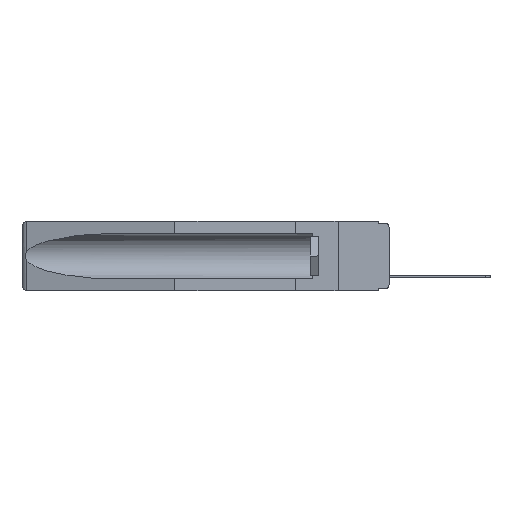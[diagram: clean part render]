
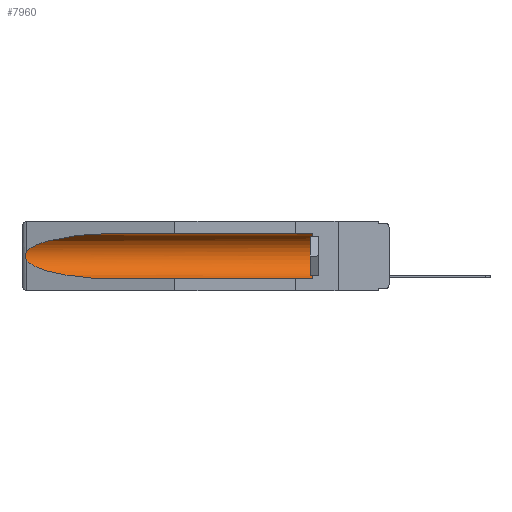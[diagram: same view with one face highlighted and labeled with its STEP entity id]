
A CAD part, left-side view. The second image highlights one B-rep face of the part: STEP entity #7960.
In plain terms, the highlighted cylindrical face has radius 2.857 mm (diameter 5.715 mm), a partial arc.
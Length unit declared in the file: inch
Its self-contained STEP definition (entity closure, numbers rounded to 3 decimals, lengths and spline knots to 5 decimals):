
#289 = FACE_OUTER_BOUND ( 'NONE', #15838, .T. ) ;
#311 = ORIENTED_EDGE ( 'NONE', *, *, #8183, .T. ) ;
#1156 = VERTEX_POINT ( 'NONE', #9793 ) ;
#1396 = CARTESIAN_POINT ( 'NONE',  ( 0.155, -0.30754, -0.1715 ) ) ;
#2450 = LINE ( 'NONE', #23616, #7621 ) ;
#2835 = CARTESIAN_POINT ( 'NONE',  ( 0.26597, 1.5296, -0.19026 ) ) ;
#3096 = CARTESIAN_POINT ( 'NONE',  ( 0.2675, 1.53308, -0.17534 ) ) ;
#3398 = ORIENTED_EDGE ( 'NONE', *, *, #13188, .T. ) ;
#4420 = CARTESIAN_POINT ( 'NONE',  ( 0.155, -0.30754, -0.059 ) ) ;
#4625 = CARTESIAN_POINT ( 'NONE',  ( 0.26537, 1.52718, -0.14972 ) ) ;
#4921 = CARTESIAN_POINT ( 'NONE',  ( 0.26537, 1.52718, -0.19328 ) ) ;
#5220 = ORIENTED_EDGE ( 'NONE', *, *, #23578, .T. ) ;
#5652 = VERTEX_POINT ( 'NONE', #22258 ) ;
#5661 =( BOUNDED_CURVE ( )  B_SPLINE_CURVE ( 3, ( #4921, #11117, #21182, #19028 ),
 .UNSPECIFIED., .F., .F. ) 
 B_SPLINE_CURVE_WITH_KNOTS ( ( 4, 4 ),
 ( 0.1948, 1.5708 ),
 .UNSPECIFIED. ) 
 CURVE ( )  GEOMETRIC_REPRESENTATION_ITEM ( )  RATIONAL_B_SPLINE_CURVE ( ( 1., 0.848, 0.848, 1. ) ) 
 REPRESENTATION_ITEM ( '' )  );
#6279 = ORIENTED_EDGE ( 'NONE', *, *, #16529, .T. ) ;
#7621 = VECTOR ( 'NONE', #11258, 39.37008 ) ;
#7960 = ADVANCED_FACE ( 'NONE', ( #289 ), #21105, .F. ) ;
#8183 = EDGE_CURVE ( 'NONE', #21654, #1156, #9186, .T. ) ;
#8205 = DIRECTION ( 'NONE',  ( 0., 0., 1. ) ) ;
#9159 = VERTEX_POINT ( 'NONE', #10405 ) ;
#9186 = LINE ( 'NONE', #4420, #14604 ) ;
#9357 = CARTESIAN_POINT ( 'NONE',  ( 0.2673, 1.5327, -0.16383 ) ) ;
#9793 = CARTESIAN_POINT ( 'NONE',  ( 0.155, 1.07973, -0.059 ) ) ;
#10405 = CARTESIAN_POINT ( 'NONE',  ( 0.155, 0.126, -0.284 ) ) ;
#10463 =( BOUNDED_CURVE ( )  B_SPLINE_CURVE ( 3, ( #15393, #19427, #17081, #25401 ),
 .UNSPECIFIED., .F., .F. ) 
 B_SPLINE_CURVE_WITH_KNOTS ( ( 4, 4 ),
 ( 4.71239, 6.08839 ),
 .UNSPECIFIED. ) 
 CURVE ( )  GEOMETRIC_REPRESENTATION_ITEM ( )  RATIONAL_B_SPLINE_CURVE ( ( 1., 0.848, 0.848, 1. ) ) 
 REPRESENTATION_ITEM ( '' )  );
#11016 = CARTESIAN_POINT ( 'NONE',  ( 0.26655, 1.53094, -0.18657 ) ) ;
#11117 = CARTESIAN_POINT ( 'NONE',  ( 0.25451, 1.48313, -0.24835 ) ) ;
#11258 = DIRECTION ( 'NONE',  ( 0., 1., 0. ) ) ;
#11755 = DIRECTION ( 'NONE',  ( 0., 0., 1. ) ) ;
#12535 = CIRCLE ( 'NONE', #20745, 0.1125 ) ;
#13171 = EDGE_CURVE ( 'NONE', #9159, #5652, #2450, .T. ) ;
#13188 = EDGE_CURVE ( 'NONE', #1156, #21971, #10463, .T. ) ;
#13197 = CARTESIAN_POINT ( 'NONE',  ( 0.2673, 1.53269, -0.17917 ) ) ;
#13644 = ORIENTED_EDGE ( 'NONE', *, *, #22303, .T. ) ;
#14483 = DIRECTION ( 'NONE',  ( 0., 1., 0. ) ) ;
#14486 = CARTESIAN_POINT ( 'NONE',  ( 0.155, 0.126, -0.1715 ) ) ;
#14604 = VECTOR ( 'NONE', #14483, 39.37008 ) ;
#15393 = CARTESIAN_POINT ( 'NONE',  ( 0.155, 1.07973, -0.059 ) ) ;
#15789 = DIRECTION ( 'NONE',  ( 0., 1., 0. ) ) ;
#15838 = EDGE_LOOP ( 'NONE', ( #3398, #6279, #5220, #25725, #13644, #311 ) ) ;
#16035 = B_SPLINE_CURVE_WITH_KNOTS ( 'NONE', 3,
 ( #19454, #19551, #25792, #9357, #25702, #3096, #13197, #11016, #2835, #23732 ),
 .UNSPECIFIED., .F., .F.,
 ( 4, 2, 2, 2, 4 ),
 ( 0., 0.00029, 0.00058, 0.00087, 0.00117 ),
 .UNSPECIFIED. ) ;
#16529 = EDGE_CURVE ( 'NONE', #21971, #24769, #16035, .T. ) ;
#17081 = CARTESIAN_POINT ( 'NONE',  ( 0.25451, 1.48313, -0.09465 ) ) ;
#19028 = CARTESIAN_POINT ( 'NONE',  ( 0.155, 1.07973, -0.284 ) ) ;
#19427 = CARTESIAN_POINT ( 'NONE',  ( 0.21114, 1.30732, -0.059 ) ) ;
#19454 = CARTESIAN_POINT ( 'NONE',  ( 0.26537, 1.52718, -0.14972 ) ) ;
#19551 = CARTESIAN_POINT ( 'NONE',  ( 0.26597, 1.52961, -0.15275 ) ) ;
#20411 = DIRECTION ( 'NONE',  ( 0., -1., 0. ) ) ;
#20745 = AXIS2_PLACEMENT_3D ( 'NONE', #14486, #20411, #8205 ) ;
#21105 = CYLINDRICAL_SURFACE ( 'NONE', #24361, 0.1125 ) ;
#21182 = CARTESIAN_POINT ( 'NONE',  ( 0.21114, 1.30732, -0.284 ) ) ;
#21654 = VERTEX_POINT ( 'NONE', #26331 ) ;
#21971 = VERTEX_POINT ( 'NONE', #4625 ) ;
#22258 = CARTESIAN_POINT ( 'NONE',  ( 0.155, 1.07973, -0.284 ) ) ;
#22303 = EDGE_CURVE ( 'NONE', #9159, #21654, #12535, .T. ) ;
#23578 = EDGE_CURVE ( 'NONE', #24769, #5652, #5661, .T. ) ;
#23616 = CARTESIAN_POINT ( 'NONE',  ( 0.155, -0.30754, -0.284 ) ) ;
#23732 = CARTESIAN_POINT ( 'NONE',  ( 0.26537, 1.52718, -0.19328 ) ) ;
#24361 = AXIS2_PLACEMENT_3D ( 'NONE', #1396, #15789, #11755 ) ;
#24769 = VERTEX_POINT ( 'NONE', #24780 ) ;
#24780 = CARTESIAN_POINT ( 'NONE',  ( 0.26537, 1.52718, -0.19328 ) ) ;
#25401 = CARTESIAN_POINT ( 'NONE',  ( 0.26537, 1.52718, -0.14972 ) ) ;
#25702 = CARTESIAN_POINT ( 'NONE',  ( 0.2675, 1.53308, -0.16763 ) ) ;
#25725 = ORIENTED_EDGE ( 'NONE', *, *, #13171, .F. ) ;
#25792 = CARTESIAN_POINT ( 'NONE',  ( 0.26654, 1.53092, -0.15636 ) ) ;
#26331 = CARTESIAN_POINT ( 'NONE',  ( 0.155, 0.126, -0.059 ) ) ;
